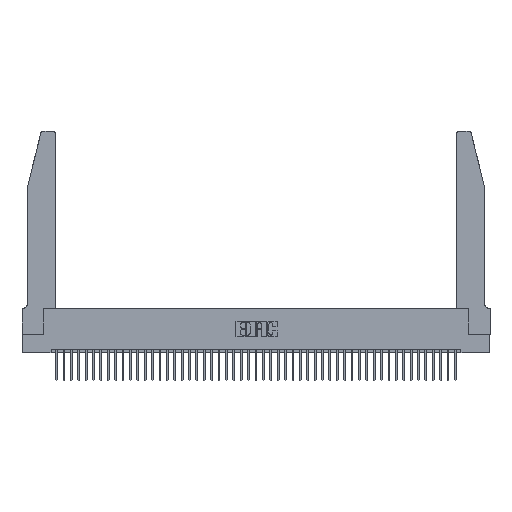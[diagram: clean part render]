
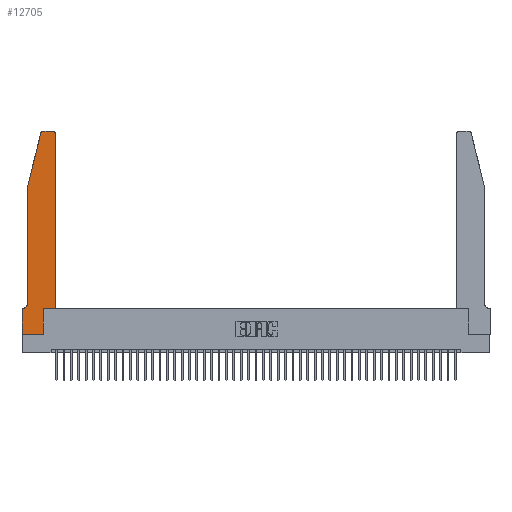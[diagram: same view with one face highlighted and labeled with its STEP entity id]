
A CAD part, top view. The second image highlights one B-rep face of the part: STEP entity #12705.
In plain terms, the highlighted planar face has unit normal (0, 0, 1).
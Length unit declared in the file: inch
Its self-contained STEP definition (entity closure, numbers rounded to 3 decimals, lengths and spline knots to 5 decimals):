
#266 = AXIS2_PLACEMENT_3D ( 'NONE', #22823, #1396, #26390 ) ;
#1396 = DIRECTION ( 'NONE',  ( 0., 0., 1. ) ) ;
#1736 = FACE_OUTER_BOUND ( 'NONE', #19212, .T. ) ;
#3224 = CIRCLE ( 'NONE', #8863, 0.03 ) ;
#3902 = ORIENTED_EDGE ( 'NONE', *, *, #21604, .T. ) ;
#3979 = VERTEX_POINT ( 'NONE', #46040 ) ;
#4736 = ORIENTED_EDGE ( 'NONE', *, *, #6880, .T. ) ;
#4829 = DIRECTION ( 'NONE',  ( 1., 0., 0. ) ) ;
#5043 = VECTOR ( 'NONE', #30345, 39.37008 ) ;
#5393 = CARTESIAN_POINT ( 'NONE',  ( 0., 0., 0.37 ) ) ;
#5421 = ORIENTED_EDGE ( 'NONE', *, *, #46150, .T. ) ;
#5525 = CARTESIAN_POINT ( 'NONE',  ( 0.0755, 0.42, 0.37 ) ) ;
#5851 = ORIENTED_EDGE ( 'NONE', *, *, #32458, .T. ) ;
#6112 = EDGE_CURVE ( 'NONE', #45227, #24269, #10090, .T. ) ;
#6227 = ORIENTED_EDGE ( 'NONE', *, *, #11127, .T. ) ;
#6562 = CARTESIAN_POINT ( 'NONE',  ( 0.0755, 2., 0.37 ) ) ;
#6880 = EDGE_CURVE ( 'NONE', #42483, #9141, #15135, .T. ) ;
#6929 = EDGE_CURVE ( 'NONE', #31601, #32434, #30746, .T. ) ;
#7129 = EDGE_CURVE ( 'NONE', #32434, #8163, #15691, .T. ) ;
#7134 = LINE ( 'NONE', #36693, #35567 ) ;
#7436 = CIRCLE ( 'NONE', #34433, 0.07 ) ;
#7476 = DIRECTION ( 'NONE',  ( 0., 0., 1. ) ) ;
#8163 = VERTEX_POINT ( 'NONE', #35685 ) ;
#8713 = DIRECTION ( 'NONE',  ( 0., 0., -1. ) ) ;
#8863 = AXIS2_PLACEMENT_3D ( 'NONE', #28818, #7476, #32413 ) ;
#9141 = VERTEX_POINT ( 'NONE', #21686 ) ;
#9726 = ORIENTED_EDGE ( 'NONE', *, *, #7129, .T. ) ;
#10090 = LINE ( 'NONE', #6562, #30200 ) ;
#11127 = EDGE_CURVE ( 'NONE', #3979, #42483, #30352, .T. ) ;
#11129 = DIRECTION ( 'NONE',  ( 1., 0., 0. ) ) ;
#11146 = CARTESIAN_POINT ( 'NONE',  ( 0.0055, 0.35, 0.37 ) ) ;
#11735 = ORIENTED_EDGE ( 'NONE', *, *, #29941, .T. ) ;
#11777 = VECTOR ( 'NONE', #18649, 39.37008 ) ;
#12705 = ADVANCED_FACE ( 'NONE', ( #1736 ), #14586, .T. ) ;
#13499 = CARTESIAN_POINT ( 'NONE',  ( 0., 0.35, 0.37 ) ) ;
#13747 = LINE ( 'NONE', #31868, #39902 ) ;
#14016 = VECTOR ( 'NONE', #36247, 39.37008 ) ;
#14586 = PLANE ( 'NONE',  #36987 ) ;
#14719 = LINE ( 'NONE', #44797, #25260 ) ;
#14884 = CARTESIAN_POINT ( 'NONE',  ( 0.0755, 2., 0.37 ) ) ;
#15135 = LINE ( 'NONE', #32694, #14016 ) ;
#15691 = LINE ( 'NONE', #5393, #5043 ) ;
#16210 = CARTESIAN_POINT ( 'NONE',  ( 0.284, 2.75, 0.37 ) ) ;
#18305 = CARTESIAN_POINT ( 'NONE',  ( 0.4205, 2.75, 0.37 ) ) ;
#18649 = DIRECTION ( 'NONE',  ( -1., 0., 0. ) ) ;
#18937 = DIRECTION ( 'NONE',  ( 0., 1., 0. ) ) ;
#19212 = EDGE_LOOP ( 'NONE', ( #5851, #11735, #43998, #33050, #25380, #45851, #9726, #31943, #3902, #6227, #4736, #5421 ) ) ;
#19765 = VECTOR ( 'NONE', #4829, 39.37008 ) ;
#20510 = CARTESIAN_POINT ( 'NONE',  ( 0.2865, 0., 0.37 ) ) ;
#21099 = VERTEX_POINT ( 'NONE', #16210 ) ;
#21417 = DIRECTION ( 'NONE',  ( 1., 0., 0. ) ) ;
#21604 = EDGE_CURVE ( 'NONE', #25893, #3979, #7134, .T. ) ;
#21686 = CARTESIAN_POINT ( 'NONE',  ( 0.4505, 2.72, 0.37 ) ) ;
#22823 = CARTESIAN_POINT ( 'NONE',  ( 0.284, 2.72, 0.37 ) ) ;
#23516 = DIRECTION ( 'NONE',  ( 0., -1., 0. ) ) ;
#24269 = VERTEX_POINT ( 'NONE', #14884 ) ;
#25260 = VECTOR ( 'NONE', #23516, 39.37008 ) ;
#25380 = ORIENTED_EDGE ( 'NONE', *, *, #28214, .T. ) ;
#25893 = VERTEX_POINT ( 'NONE', #20510 ) ;
#26390 = DIRECTION ( 'NONE',  ( 1., 0., 0. ) ) ;
#28214 = EDGE_CURVE ( 'NONE', #28973, #31601, #7436, .T. ) ;
#28818 = CARTESIAN_POINT ( 'NONE',  ( 0.4205, 2.72, 0.37 ) ) ;
#28889 = CARTESIAN_POINT ( 'NONE',  ( 0., 0.35, 0.37 ) ) ;
#28973 = VERTEX_POINT ( 'NONE', #5525 ) ;
#29457 = LINE ( 'NONE', #38543, #37813 ) ;
#29941 = EDGE_CURVE ( 'NONE', #21099, #45227, #32927, .T. ) ;
#30054 = CARTESIAN_POINT ( 'NONE',  ( 0.0055, 0.42, 0.37 ) ) ;
#30179 = CARTESIAN_POINT ( 'NONE',  ( 0.4505, 0.35, 0.37 ) ) ;
#30200 = VECTOR ( 'NONE', #31493, 39.37008 ) ;
#30345 = DIRECTION ( 'NONE',  ( 0., -1., 0. ) ) ;
#30352 = LINE ( 'NONE', #40359, #19765 ) ;
#30746 = LINE ( 'NONE', #36410, #11777 ) ;
#31493 = DIRECTION ( 'NONE',  ( -0.239, -0.971, 0. ) ) ;
#31601 = VERTEX_POINT ( 'NONE', #11146 ) ;
#31868 = CARTESIAN_POINT ( 'NONE',  ( 0., 0., 0.37 ) ) ;
#31943 = ORIENTED_EDGE ( 'NONE', *, *, #34528, .T. ) ;
#32413 = DIRECTION ( 'NONE',  ( 1., 0., 0. ) ) ;
#32434 = VERTEX_POINT ( 'NONE', #13499 ) ;
#32458 = EDGE_CURVE ( 'NONE', #39968, #21099, #29457, .T. ) ;
#32488 = DIRECTION ( 'NONE',  ( 0., 0., 1. ) ) ;
#32694 = CARTESIAN_POINT ( 'NONE',  ( 0.4505, 0.35, 0.37 ) ) ;
#32927 = CIRCLE ( 'NONE', #266, 0.03 ) ;
#33050 = ORIENTED_EDGE ( 'NONE', *, *, #35817, .T. ) ;
#33658 = DIRECTION ( 'NONE',  ( -1., 0., 0. ) ) ;
#34433 = AXIS2_PLACEMENT_3D ( 'NONE', #30054, #8713, #33658 ) ;
#34528 = EDGE_CURVE ( 'NONE', #8163, #25893, #13747, .T. ) ;
#35567 = VECTOR ( 'NONE', #18937, 39.37008 ) ;
#35685 = CARTESIAN_POINT ( 'NONE',  ( 0., 0., 0.37 ) ) ;
#35817 = EDGE_CURVE ( 'NONE', #24269, #28973, #14719, .T. ) ;
#36247 = DIRECTION ( 'NONE',  ( 0., 1., 0. ) ) ;
#36410 = CARTESIAN_POINT ( 'NONE',  ( 0.0755, 0.35, 0.37 ) ) ;
#36693 = CARTESIAN_POINT ( 'NONE',  ( 0.2865, 0.35, 0.37 ) ) ;
#36987 = AXIS2_PLACEMENT_3D ( 'NONE', #28889, #32488, #11129 ) ;
#37813 = VECTOR ( 'NONE', #42096, 39.37008 ) ;
#38543 = CARTESIAN_POINT ( 'NONE',  ( 0.2605, 2.75, 0.37 ) ) ;
#39902 = VECTOR ( 'NONE', #21417, 39.37008 ) ;
#39968 = VERTEX_POINT ( 'NONE', #18305 ) ;
#40359 = CARTESIAN_POINT ( 'NONE',  ( 0.4505, 0.35, 0.37 ) ) ;
#42096 = DIRECTION ( 'NONE',  ( -1., 0., 0. ) ) ;
#42483 = VERTEX_POINT ( 'NONE', #30179 ) ;
#43998 = ORIENTED_EDGE ( 'NONE', *, *, #6112, .T. ) ;
#44718 = CARTESIAN_POINT ( 'NONE',  ( 0.25487, 2.72718, 0.37 ) ) ;
#44797 = CARTESIAN_POINT ( 'NONE',  ( 0.0755, 2., 0.37 ) ) ;
#45227 = VERTEX_POINT ( 'NONE', #44718 ) ;
#45851 = ORIENTED_EDGE ( 'NONE', *, *, #6929, .T. ) ;
#46040 = CARTESIAN_POINT ( 'NONE',  ( 0.2865, 0.35, 0.37 ) ) ;
#46150 = EDGE_CURVE ( 'NONE', #9141, #39968, #3224, .T. ) ;
